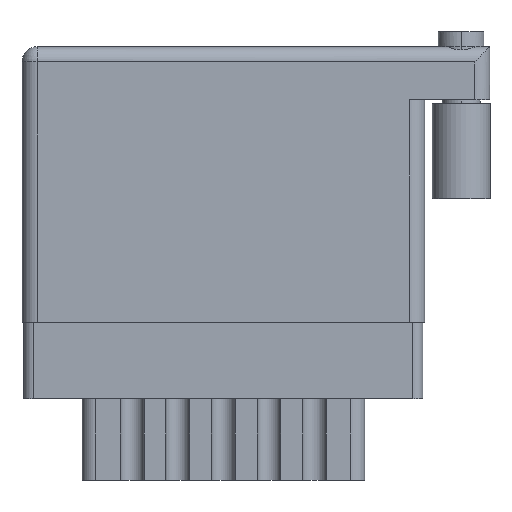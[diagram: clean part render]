
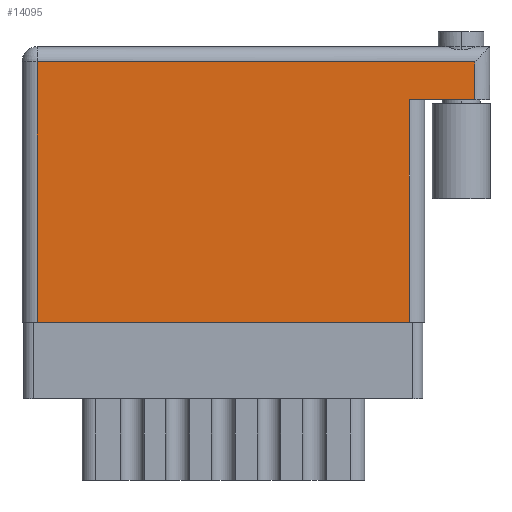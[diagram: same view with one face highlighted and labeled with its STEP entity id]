
A CAD part, front view. The second image highlights one B-rep face of the part: STEP entity #14095.
In plain terms, the highlighted face is planar.
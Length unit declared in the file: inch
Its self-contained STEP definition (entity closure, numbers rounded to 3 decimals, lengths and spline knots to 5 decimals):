
#278 = ORIENTED_EDGE ( 'NONE', *, *, #11623, .T. ) ;
#703 = LINE ( 'NONE', #15728, #12518 ) ;
#1401 = DIRECTION ( 'NONE',  ( 0., -1., 0. ) ) ;
#1610 = LINE ( 'NONE', #14474, #11103 ) ;
#1670 = CARTESIAN_POINT ( 'NONE',  ( 0.05, 0., 0. ) ) ;
#1852 = AXIS2_PLACEMENT_3D ( 'NONE', #13280, #3224, #10124 ) ;
#2070 = EDGE_CURVE ( 'NONE', #20715, #4197, #1610, .T. ) ;
#2516 = EDGE_CURVE ( 'NONE', #4197, #17361, #21056, .T. ) ;
#2886 = DIRECTION ( 'NONE',  ( -1., 0., 0. ) ) ;
#2966 = CARTESIAN_POINT ( 'NONE',  ( 1.275, 0.731, 0. ) ) ;
#3154 = CARTESIAN_POINT ( 'NONE',  ( 1.489, 0.856, 0. ) ) ;
#3224 = DIRECTION ( 'NONE',  ( 0., 0., -1. ) ) ;
#4197 = VERTEX_POINT ( 'NONE', #1670 ) ;
#4543 = VERTEX_POINT ( 'NONE', #3154 ) ;
#4796 = VECTOR ( 'NONE', #2886, 39.37008 ) ;
#6244 = ORIENTED_EDGE ( 'NONE', *, *, #19222, .T. ) ;
#6321 = DIRECTION ( 'NONE',  ( 0., 1., 0. ) ) ;
#7006 = ORIENTED_EDGE ( 'NONE', *, *, #8688, .T. ) ;
#7732 = LINE ( 'NONE', #11209, #4796 ) ;
#7949 = CARTESIAN_POINT ( 'NONE',  ( 0., 0., 0. ) ) ;
#8171 = DIRECTION ( 'NONE',  ( 1., 0., 0. ) ) ;
#8688 = EDGE_CURVE ( 'NONE', #4543, #20715, #7732, .T. ) ;
#9393 = VERTEX_POINT ( 'NONE', #11896 ) ;
#10124 = DIRECTION ( 'NONE',  ( -1., 0., 0. ) ) ;
#10792 = ORIENTED_EDGE ( 'NONE', *, *, #11628, .F. ) ;
#11103 = VECTOR ( 'NONE', #1401, 39.37008 ) ;
#11209 = CARTESIAN_POINT ( 'NONE',  ( 0., 0.856, 0. ) ) ;
#11623 = EDGE_CURVE ( 'NONE', #9393, #4543, #18843, .T. ) ;
#11628 = EDGE_CURVE ( 'NONE', #9393, #14537, #703, .T. ) ;
#11695 = ORIENTED_EDGE ( 'NONE', *, *, #2070, .T. ) ;
#11818 = VECTOR ( 'NONE', #8171, 39.37008 ) ;
#11844 = ORIENTED_EDGE ( 'NONE', *, *, #2516, .T. ) ;
#11896 = CARTESIAN_POINT ( 'NONE',  ( 1.489, 0.731, 0. ) ) ;
#12235 = CARTESIAN_POINT ( 'NONE',  ( 0.05, 0.856, 0. ) ) ;
#12518 = VECTOR ( 'NONE', #13782, 39.37008 ) ;
#13280 = CARTESIAN_POINT ( 'NONE',  ( 0., 0.906, 0. ) ) ;
#13782 = DIRECTION ( 'NONE',  ( -1., 0., 0. ) ) ;
#14095 = ADVANCED_FACE ( 'NONE', ( #16834 ), #16297, .F. ) ;
#14474 = CARTESIAN_POINT ( 'NONE',  ( 0.05, 0., 0. ) ) ;
#14537 = VERTEX_POINT ( 'NONE', #16495 ) ;
#15595 = EDGE_LOOP ( 'NONE', ( #11844, #6244, #10792, #278, #7006, #11695 ) ) ;
#15728 = CARTESIAN_POINT ( 'NONE',  ( 1.539, 0.731, 0. ) ) ;
#15844 = VECTOR ( 'NONE', #6321, 39.37008 ) ;
#16297 = PLANE ( 'NONE',  #1852 ) ;
#16495 = CARTESIAN_POINT ( 'NONE',  ( 1.275, 0.731, 0. ) ) ;
#16834 = FACE_OUTER_BOUND ( 'NONE', #15595, .T. ) ;
#17330 = DIRECTION ( 'NONE',  ( 0., 1., 0. ) ) ;
#17340 = VECTOR ( 'NONE', #17330, 39.37008 ) ;
#17361 = VERTEX_POINT ( 'NONE', #19307 ) ;
#18082 = LINE ( 'NONE', #2966, #15844 ) ;
#18843 = LINE ( 'NONE', #20708, #17340 ) ;
#19222 = EDGE_CURVE ( 'NONE', #17361, #14537, #18082, .T. ) ;
#19307 = CARTESIAN_POINT ( 'NONE',  ( 1.275, 0., 0. ) ) ;
#20708 = CARTESIAN_POINT ( 'NONE',  ( 1.489, 0.906, 0. ) ) ;
#20715 = VERTEX_POINT ( 'NONE', #12235 ) ;
#21056 = LINE ( 'NONE', #7949, #11818 ) ;
